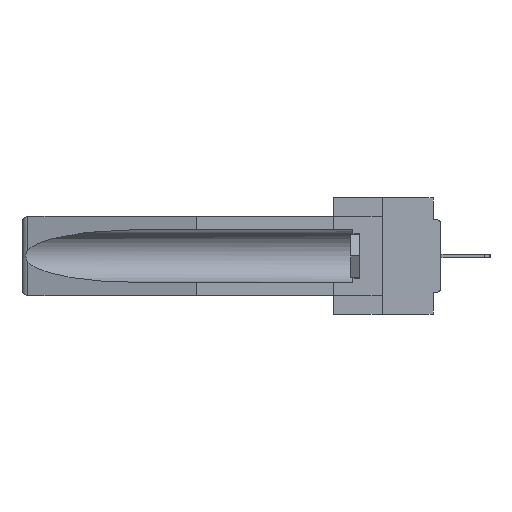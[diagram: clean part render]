
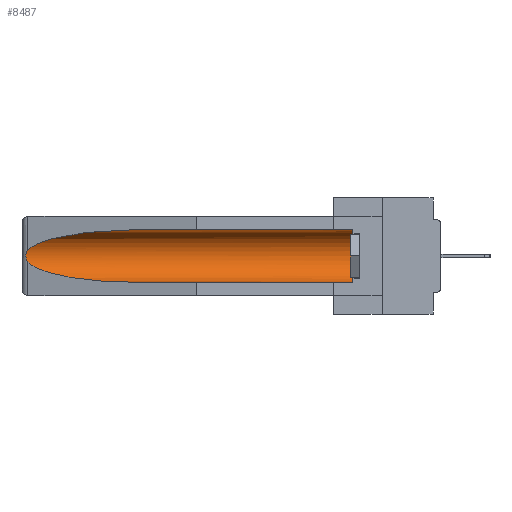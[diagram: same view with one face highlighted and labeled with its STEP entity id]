
A CAD part, left-side view. The second image highlights one B-rep face of the part: STEP entity #8487.
In plain terms, the highlighted cylindrical face has radius 2.857 mm (diameter 5.715 mm), a partial arc.
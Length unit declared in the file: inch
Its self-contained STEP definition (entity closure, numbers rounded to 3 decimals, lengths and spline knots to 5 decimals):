
#121 = CARTESIAN_POINT ( 'NONE',  ( 0.26597, 1.5296, -0.19026 ) ) ;
#259 = DIRECTION ( 'NONE',  ( 0., 1., 0. ) ) ;
#332 = CARTESIAN_POINT ( 'NONE',  ( 0.155, 1.07973, -0.059 ) ) ;
#557 = AXIS2_PLACEMENT_3D ( 'NONE', #18945, #259, #16325 ) ;
#674 = EDGE_CURVE ( 'NONE', #32819, #9354, #7222, .T. ) ;
#2865 = VERTEX_POINT ( 'NONE', #16222 ) ;
#3132 = CARTESIAN_POINT ( 'NONE',  ( 0.21114, 1.30732, -0.059 ) ) ;
#4552 = CARTESIAN_POINT ( 'NONE',  ( 0.155, -0.30754, -0.284 ) ) ;
#5555 = CARTESIAN_POINT ( 'NONE',  ( 0.26597, 1.52961, -0.15275 ) ) ;
#5725 = CARTESIAN_POINT ( 'NONE',  ( 0.155, 1.07973, -0.059 ) ) ;
#5870 = CARTESIAN_POINT ( 'NONE',  ( 0.26537, 1.52718, -0.14972 ) ) ;
#6654 = ORIENTED_EDGE ( 'NONE', *, *, #19222, .T. ) ;
#7027 = AXIS2_PLACEMENT_3D ( 'NONE', #28724, #12944, #31354 ) ;
#7222 = LINE ( 'NONE', #4552, #33541 ) ;
#7426 = CARTESIAN_POINT ( 'NONE',  ( 0.26537, 1.52718, -0.14972 ) ) ;
#8306 = DIRECTION ( 'NONE',  ( 0., 1., 0. ) ) ;
#8487 = ADVANCED_FACE ( 'NONE', ( #13502 ), #26674, .F. ) ;
#9354 = VERTEX_POINT ( 'NONE', #14129 ) ;
#9907 = ORIENTED_EDGE ( 'NONE', *, *, #25089, .T. ) ;
#10352 = ORIENTED_EDGE ( 'NONE', *, *, #21433, .T. ) ;
#10414 = VERTEX_POINT ( 'NONE', #5725 ) ;
#10628 = VERTEX_POINT ( 'NONE', #11721 ) ;
#10879 = CARTESIAN_POINT ( 'NONE',  ( 0.2673, 1.5327, -0.16383 ) ) ;
#11433 = VERTEX_POINT ( 'NONE', #7426 ) ;
#11721 = CARTESIAN_POINT ( 'NONE',  ( 0.26537, 1.52718, -0.19328 ) ) ;
#11835 = CARTESIAN_POINT ( 'NONE',  ( 0.25451, 1.48313, -0.24835 ) ) ;
#11911 = EDGE_LOOP ( 'NONE', ( #9907, #10352, #26854, #19002, #6654, #16828 ) ) ;
#12242 = B_SPLINE_CURVE_WITH_KNOTS ( 'NONE', 3,
 ( #18700, #5555, #26668, #10879, #29325, #13547, #31925, #16196, #121, #18817 ),
 .UNSPECIFIED., .F., .F.,
 ( 4, 2, 2, 2, 4 ),
 ( 0., 0.00029, 0.00058, 0.00087, 0.00117 ),
 .UNSPECIFIED. ) ;
#12944 = DIRECTION ( 'NONE',  ( 0., -1., 0. ) ) ;
#12980 = CIRCLE ( 'NONE', #7027, 0.1125 ) ;
#13502 = FACE_OUTER_BOUND ( 'NONE', #11911, .T. ) ;
#13547 = CARTESIAN_POINT ( 'NONE',  ( 0.2675, 1.53308, -0.17534 ) ) ;
#14129 = CARTESIAN_POINT ( 'NONE',  ( 0.155, 1.07973, -0.284 ) ) ;
#14752 = CARTESIAN_POINT ( 'NONE',  ( 0.155, 1.07973, -0.284 ) ) ;
#16196 = CARTESIAN_POINT ( 'NONE',  ( 0.26655, 1.53094, -0.18657 ) ) ;
#16222 = CARTESIAN_POINT ( 'NONE',  ( 0.155, 0.126, -0.059 ) ) ;
#16325 = DIRECTION ( 'NONE',  ( 0., 0., 1. ) ) ;
#16828 = ORIENTED_EDGE ( 'NONE', *, *, #19023, .T. ) ;
#17006 = EDGE_CURVE ( 'NONE', #10628, #9354, #26376, .T. ) ;
#18700 = CARTESIAN_POINT ( 'NONE',  ( 0.26537, 1.52718, -0.14972 ) ) ;
#18738 = VECTOR ( 'NONE', #22497, 39.37008 ) ;
#18817 = CARTESIAN_POINT ( 'NONE',  ( 0.26537, 1.52718, -0.19328 ) ) ;
#18945 = CARTESIAN_POINT ( 'NONE',  ( 0.155, -0.30754, -0.1715 ) ) ;
#19002 = ORIENTED_EDGE ( 'NONE', *, *, #674, .F. ) ;
#19023 = EDGE_CURVE ( 'NONE', #2865, #10414, #33549, .T. ) ;
#19222 = EDGE_CURVE ( 'NONE', #32819, #2865, #12980, .T. ) ;
#21433 = EDGE_CURVE ( 'NONE', #11433, #10628, #12242, .T. ) ;
#21657 = CARTESIAN_POINT ( 'NONE',  ( 0.25451, 1.48313, -0.09465 ) ) ;
#22497 = DIRECTION ( 'NONE',  ( 0., 1., 0. ) ) ;
#24705 = CARTESIAN_POINT ( 'NONE',  ( 0.155, 0.126, -0.284 ) ) ;
#25040 = CARTESIAN_POINT ( 'NONE',  ( 0.155, -0.30754, -0.059 ) ) ;
#25089 = EDGE_CURVE ( 'NONE', #10414, #11433, #32772, .T. ) ;
#25205 = CARTESIAN_POINT ( 'NONE',  ( 0.26537, 1.52718, -0.19328 ) ) ;
#26376 =( BOUNDED_CURVE ( )  B_SPLINE_CURVE ( 3, ( #25205, #11835, #30518, #14752 ),
 .UNSPECIFIED., .F., .F. ) 
 B_SPLINE_CURVE_WITH_KNOTS ( ( 4, 4 ),
 ( 0.1948, 1.5708 ),
 .UNSPECIFIED. ) 
 CURVE ( )  GEOMETRIC_REPRESENTATION_ITEM ( )  RATIONAL_B_SPLINE_CURVE ( ( 1., 0.848, 0.848, 1. ) ) 
 REPRESENTATION_ITEM ( '' )  );
#26668 = CARTESIAN_POINT ( 'NONE',  ( 0.26654, 1.53092, -0.15636 ) ) ;
#26674 = CYLINDRICAL_SURFACE ( 'NONE', #557, 0.1125 ) ;
#26854 = ORIENTED_EDGE ( 'NONE', *, *, #17006, .T. ) ;
#28724 = CARTESIAN_POINT ( 'NONE',  ( 0.155, 0.126, -0.1715 ) ) ;
#29325 = CARTESIAN_POINT ( 'NONE',  ( 0.2675, 1.53308, -0.16763 ) ) ;
#30518 = CARTESIAN_POINT ( 'NONE',  ( 0.21114, 1.30732, -0.284 ) ) ;
#31354 = DIRECTION ( 'NONE',  ( 0., 0., 1. ) ) ;
#31925 = CARTESIAN_POINT ( 'NONE',  ( 0.2673, 1.53269, -0.17917 ) ) ;
#32772 =( BOUNDED_CURVE ( )  B_SPLINE_CURVE ( 3, ( #332, #3132, #21657, #5870 ),
 .UNSPECIFIED., .F., .F. ) 
 B_SPLINE_CURVE_WITH_KNOTS ( ( 4, 4 ),
 ( 4.71239, 6.08839 ),
 .UNSPECIFIED. ) 
 CURVE ( )  GEOMETRIC_REPRESENTATION_ITEM ( )  RATIONAL_B_SPLINE_CURVE ( ( 1., 0.848, 0.848, 1. ) ) 
 REPRESENTATION_ITEM ( '' )  );
#32819 = VERTEX_POINT ( 'NONE', #24705 ) ;
#33541 = VECTOR ( 'NONE', #8306, 39.37008 ) ;
#33549 = LINE ( 'NONE', #25040, #18738 ) ;
